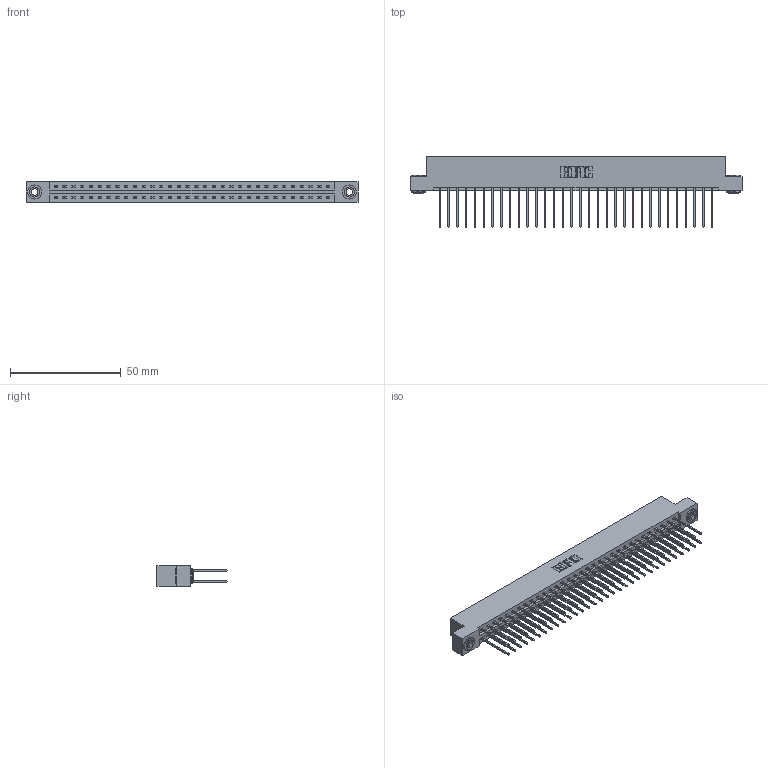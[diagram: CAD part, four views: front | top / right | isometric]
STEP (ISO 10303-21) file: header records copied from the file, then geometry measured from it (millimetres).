
FILE_DESCRIPTION (( 'STEP AP203' ), '1' );
FILE_NAME ('387-064-542-203.STEP', '2018-09-21T07:43:02', ( '' ), ( '' ), 'SwSTEP 2.0', 'SolidWorks 2016', '' );
FILE_SCHEMA (( 'CONFIG_CONTROL_DESIGN' ));
Length unit declared in the file: inch
Products named in the file (4): 387-064-542-203; 337 Part_Flush Mounting Lugs - 0.156 Dia-TH; 345-292-001_345-293-142; 345-250-002_345-250-002-102
Assembly tree (67 placements, depth 2):
  387-064-542-203
    337 Part_Flush Mounting Lugs - 0.156 Dia-TH
    345-292-001_345-293-142  x64
    345-250-002_345-250-002-102  x2
Bounding box: 149.81 x 31.63 x 9.4 mm (x, y, z)
Volume: 15972.7 mm3; surface area: 19671.8 mm2
Topology: 67 solids, 67 shells, 3608 faces, 10691 edges, 7038 vertices
Faces by surface type: plane 2512, cylinder 1088, cone 8
Entity records: 26772 total; most frequent: CARTESIAN_POINT 4493, ORIENTED_EDGE 4422, DIRECTION 3873, EDGE_CURVE 2211, LINE 2059, VECTOR 2059, VERTEX_POINT 1470, AXIS2_PLACEMENT_3D 907
